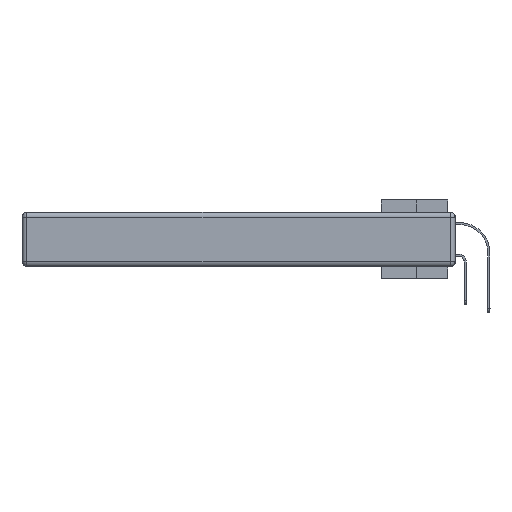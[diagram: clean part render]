
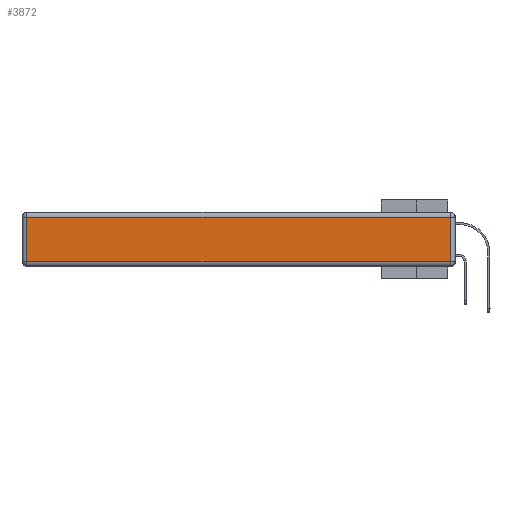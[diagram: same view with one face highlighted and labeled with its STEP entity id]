
A CAD part, left-side view. The second image highlights one B-rep face of the part: STEP entity #3872.
In plain terms, the highlighted planar face has unit normal (-1, 0, 0).
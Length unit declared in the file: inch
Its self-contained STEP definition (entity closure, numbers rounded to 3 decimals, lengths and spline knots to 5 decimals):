
#428 = LINE ( 'NONE', #6645, #9746 ) ;
#757 = DIRECTION ( 'NONE',  ( 0., 1., 0. ) ) ;
#2279 = DIRECTION ( 'NONE',  ( -1., 0., 0. ) ) ;
#3872 = ADVANCED_FACE ( 'NONE', ( #17088 ), #17733, .T. ) ;
#4183 = LINE ( 'NONE', #24565, #39403 ) ;
#5431 = CARTESIAN_POINT ( 'NONE',  ( 0., 2.72, -0.343 ) ) ;
#6645 = CARTESIAN_POINT ( 'NONE',  ( 0., 0., -0.313 ) ) ;
#7856 = CARTESIAN_POINT ( 'NONE',  ( 0., 0.03, -0.03 ) ) ;
#9746 = VECTOR ( 'NONE', #22748, 39.37008 ) ;
#10210 = EDGE_CURVE ( 'NONE', #32296, #13481, #4183, .T. ) ;
#13481 = VERTEX_POINT ( 'NONE', #20046 ) ;
#13616 = LINE ( 'NONE', #13835, #17684 ) ;
#13835 = CARTESIAN_POINT ( 'NONE',  ( 0., 0.03, -0.343 ) ) ;
#14899 = AXIS2_PLACEMENT_3D ( 'NONE', #30796, #2279, #34837 ) ;
#15928 = EDGE_LOOP ( 'NONE', ( #24536, #24806, #35482, #28345 ) ) ;
#16110 = VERTEX_POINT ( 'NONE', #29953 ) ;
#17088 = FACE_OUTER_BOUND ( 'NONE', #15928, .T. ) ;
#17684 = VECTOR ( 'NONE', #30110, 39.37008 ) ;
#17733 = PLANE ( 'NONE',  #14899 ) ;
#18984 = EDGE_CURVE ( 'NONE', #20477, #16110, #428, .T. ) ;
#20046 = CARTESIAN_POINT ( 'NONE',  ( 0., 2.72, -0.03 ) ) ;
#20477 = VERTEX_POINT ( 'NONE', #40290 ) ;
#22748 = DIRECTION ( 'NONE',  ( 0., -1., 0. ) ) ;
#24536 = ORIENTED_EDGE ( 'NONE', *, *, #18984, .T. ) ;
#24565 = CARTESIAN_POINT ( 'NONE',  ( 0., 2.75, -0.03 ) ) ;
#24806 = ORIENTED_EDGE ( 'NONE', *, *, #30312, .T. ) ;
#28345 = ORIENTED_EDGE ( 'NONE', *, *, #33938, .T. ) ;
#28587 = LINE ( 'NONE', #5431, #34906 ) ;
#29953 = CARTESIAN_POINT ( 'NONE',  ( 0., 0.03, -0.313 ) ) ;
#30110 = DIRECTION ( 'NONE',  ( 0., 0., 1. ) ) ;
#30312 = EDGE_CURVE ( 'NONE', #16110, #32296, #13616, .T. ) ;
#30796 = CARTESIAN_POINT ( 'NONE',  ( 0., 0., -0.343 ) ) ;
#32296 = VERTEX_POINT ( 'NONE', #7856 ) ;
#33938 = EDGE_CURVE ( 'NONE', #13481, #20477, #28587, .T. ) ;
#34837 = DIRECTION ( 'NONE',  ( 0., 0., 1. ) ) ;
#34906 = VECTOR ( 'NONE', #41652, 39.37008 ) ;
#35482 = ORIENTED_EDGE ( 'NONE', *, *, #10210, .T. ) ;
#39403 = VECTOR ( 'NONE', #757, 39.37008 ) ;
#40290 = CARTESIAN_POINT ( 'NONE',  ( 0., 2.72, -0.313 ) ) ;
#41652 = DIRECTION ( 'NONE',  ( 0., 0., -1. ) ) ;
